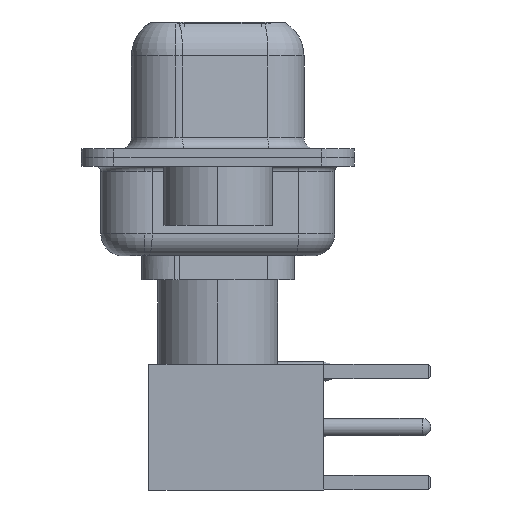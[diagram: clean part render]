
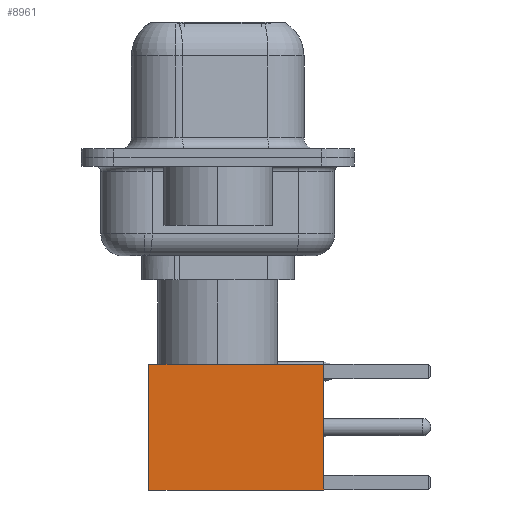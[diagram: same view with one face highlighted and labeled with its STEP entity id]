
A CAD part, left-side view. The second image highlights one B-rep face of the part: STEP entity #8961.
In plain terms, the highlighted face is planar.
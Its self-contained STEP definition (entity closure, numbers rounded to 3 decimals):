
#98 = DIRECTION ( 'NONE',  ( -1., 0., 0. ) ) ;
#413 = PLANE ( 'NONE',  #15103 ) ;
#667 = EDGE_CURVE ( 'NONE', #17370, #4054, #18230, .T. ) ;
#2130 = DIRECTION ( 'NONE',  ( 0., 1., 0. ) ) ;
#4054 = VERTEX_POINT ( 'NONE', #19686 ) ;
#4506 = LINE ( 'NONE', #18990, #20577 ) ;
#4921 = VECTOR ( 'NONE', #19898, 1000. ) ;
#5286 = ORIENTED_EDGE ( 'NONE', *, *, #15833, .T. ) ;
#5812 = DIRECTION ( 'NONE',  ( 0., 0., 1. ) ) ;
#8647 = VERTEX_POINT ( 'NONE', #16263 ) ;
#8961 = ADVANCED_FACE ( 'NONE', ( #15011 ), #413, .T. ) ;
#9427 = LINE ( 'NONE', #9538, #10148 ) ;
#9538 = CARTESIAN_POINT ( 'NONE',  ( 0., 2.875, 8. ) ) ;
#10148 = VECTOR ( 'NONE', #98, 1000. ) ;
#10392 = EDGE_CURVE ( 'NONE', #8647, #23251, #20021, .T. ) ;
#10409 = CARTESIAN_POINT ( 'NONE',  ( -2.875, 2.875, 8. ) ) ;
#10918 = VECTOR ( 'NONE', #11095, 1000. ) ;
#11095 = DIRECTION ( 'NONE',  ( 0., 0., -1. ) ) ;
#13176 = CARTESIAN_POINT ( 'NONE',  ( 2.875, 2.875, 0. ) ) ;
#14799 = ORIENTED_EDGE ( 'NONE', *, *, #10392, .T. ) ;
#15011 = FACE_OUTER_BOUND ( 'NONE', #21034, .T. ) ;
#15103 = AXIS2_PLACEMENT_3D ( 'NONE', #13176, #2130, #5812 ) ;
#15833 = EDGE_CURVE ( 'NONE', #23251, #4054, #4506, .T. ) ;
#16263 = CARTESIAN_POINT ( 'NONE',  ( 2.875, 2.875, 8. ) ) ;
#17370 = VERTEX_POINT ( 'NONE', #10409 ) ;
#18230 = LINE ( 'NONE', #18474, #10918 ) ;
#18474 = CARTESIAN_POINT ( 'NONE',  ( -2.875, 2.875, 0. ) ) ;
#18846 = ORIENTED_EDGE ( 'NONE', *, *, #667, .F. ) ;
#18928 = ORIENTED_EDGE ( 'NONE', *, *, #19294, .F. ) ;
#18990 = CARTESIAN_POINT ( 'NONE',  ( 0., 2.875, 0. ) ) ;
#19294 = EDGE_CURVE ( 'NONE', #8647, #17370, #9427, .T. ) ;
#19674 = CARTESIAN_POINT ( 'NONE',  ( 2.875, 2.875, 0. ) ) ;
#19686 = CARTESIAN_POINT ( 'NONE',  ( -2.875, 2.875, 0. ) ) ;
#19898 = DIRECTION ( 'NONE',  ( 0., 0., -1. ) ) ;
#20021 = LINE ( 'NONE', #21728, #4921 ) ;
#20577 = VECTOR ( 'NONE', #23153, 1000. ) ;
#21034 = EDGE_LOOP ( 'NONE', ( #14799, #5286, #18846, #18928 ) ) ;
#21728 = CARTESIAN_POINT ( 'NONE',  ( 2.875, 2.875, 0. ) ) ;
#23153 = DIRECTION ( 'NONE',  ( -1., 0., 0. ) ) ;
#23251 = VERTEX_POINT ( 'NONE', #19674 ) ;
